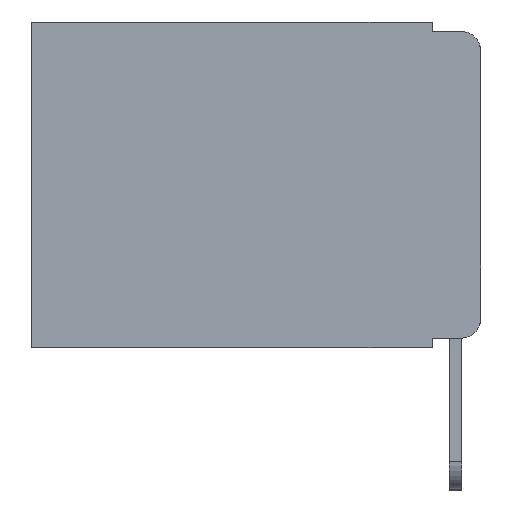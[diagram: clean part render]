
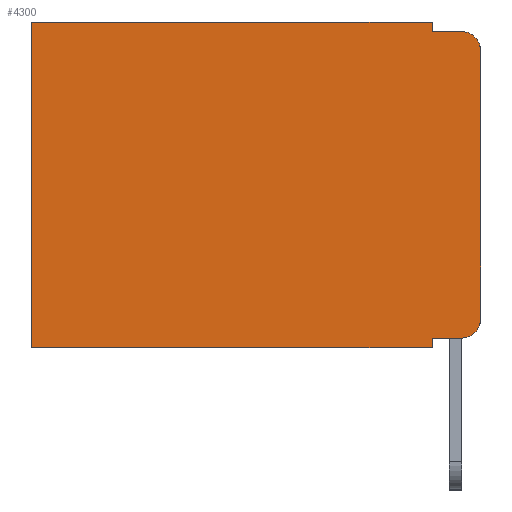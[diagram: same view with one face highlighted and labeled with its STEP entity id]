
A CAD part, left-side view. The second image highlights one B-rep face of the part: STEP entity #4300.
In plain terms, the highlighted planar face has unit normal (-1, 0, 0).
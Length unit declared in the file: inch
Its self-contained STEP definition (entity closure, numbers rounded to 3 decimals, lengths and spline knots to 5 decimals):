
#164 = EDGE_CURVE ( 'NONE', #15296, #22879, #1256, .T. ) ;
#777 = VERTEX_POINT ( 'NONE', #16168 ) ;
#849 = DIRECTION ( 'NONE',  ( 0., 0., -1. ) ) ;
#1256 = CIRCLE ( 'NONE', #5883, 0.02 ) ;
#1416 = ORIENTED_EDGE ( 'NONE', *, *, #164, .T. ) ;
#1510 = VERTEX_POINT ( 'NONE', #14155 ) ;
#1561 = ORIENTED_EDGE ( 'NONE', *, *, #21444, .F. ) ;
#1682 = DIRECTION ( 'NONE',  ( 0., 0., -1. ) ) ;
#1694 = CARTESIAN_POINT ( 'NONE',  ( 0.298, 0., -0.343 ) ) ;
#1709 = CIRCLE ( 'NONE', #3856, 0.02 ) ;
#2006 = EDGE_CURVE ( 'NONE', #1510, #4283, #5034, .T. ) ;
#2026 = VERTEX_POINT ( 'NONE', #12445 ) ;
#2494 = EDGE_CURVE ( 'NONE', #18957, #16139, #8361, .T. ) ;
#2619 = CARTESIAN_POINT ( 'NONE',  ( 0.298, 0.051, -0.333 ) ) ;
#3323 = DIRECTION ( 'NONE',  ( 0., 1., 0. ) ) ;
#3759 = CARTESIAN_POINT ( 'NONE',  ( 0.298, 0., 0. ) ) ;
#3856 = AXIS2_PLACEMENT_3D ( 'NONE', #24052, #13098, #1682 ) ;
#4224 = LINE ( 'NONE', #21386, #13761 ) ;
#4283 = VERTEX_POINT ( 'NONE', #6185 ) ;
#4300 = ADVANCED_FACE ( 'NONE', ( #16237 ), #23213, .F. ) ;
#4496 = LINE ( 'NONE', #1694, #18894 ) ;
#4603 = CARTESIAN_POINT ( 'NONE',  ( 0.298, 0.051, 0. ) ) ;
#4742 = LINE ( 'NONE', #4603, #18541 ) ;
#4749 = CARTESIAN_POINT ( 'NONE',  ( 0.298, 0.02, -0.313 ) ) ;
#4922 = EDGE_CURVE ( 'NONE', #18957, #15296, #13359, .T. ) ;
#5034 = LINE ( 'NONE', #3759, #14545 ) ;
#5145 = DIRECTION ( 'NONE',  ( 0., 0., -1. ) ) ;
#5883 = AXIS2_PLACEMENT_3D ( 'NONE', #4749, #16688, #16767 ) ;
#6026 = DIRECTION ( 'NONE',  ( 1., 0., 0. ) ) ;
#6163 = DIRECTION ( 'NONE',  ( 0., 0., -1. ) ) ;
#6185 = CARTESIAN_POINT ( 'NONE',  ( 0.298, 0.473, 0. ) ) ;
#6301 = CARTESIAN_POINT ( 'NONE',  ( 0.298, 0.02, -0.01 ) ) ;
#6323 = DIRECTION ( 'NONE',  ( 0., 1., 0. ) ) ;
#6912 = AXIS2_PLACEMENT_3D ( 'NONE', #14795, #6026, #6163 ) ;
#6964 = VECTOR ( 'NONE', #23425, 39.37008 ) ;
#7570 = LINE ( 'NONE', #10543, #6964 ) ;
#7580 = DIRECTION ( 'NONE',  ( 0., -1., 0. ) ) ;
#7673 = EDGE_CURVE ( 'NONE', #2026, #23651, #4224, .T. ) ;
#7700 = LINE ( 'NONE', #18250, #12723 ) ;
#8173 = ORIENTED_EDGE ( 'NONE', *, *, #2006, .T. ) ;
#8288 = EDGE_CURVE ( 'NONE', #16139, #19337, #4496, .T. ) ;
#8361 = LINE ( 'NONE', #8645, #17631 ) ;
#8419 = ORIENTED_EDGE ( 'NONE', *, *, #8288, .F. ) ;
#8645 = CARTESIAN_POINT ( 'NONE',  ( 0.298, 0.051, 0. ) ) ;
#8699 = CARTESIAN_POINT ( 'NONE',  ( 0.298, 0.02, -0.333 ) ) ;
#8938 = VECTOR ( 'NONE', #7580, 39.37008 ) ;
#10013 = DIRECTION ( 'NONE',  ( 0., 0., -1. ) ) ;
#10543 = CARTESIAN_POINT ( 'NONE',  ( 0.298, 0., 0. ) ) ;
#11507 = ORIENTED_EDGE ( 'NONE', *, *, #2494, .F. ) ;
#11787 = EDGE_CURVE ( 'NONE', #1510, #2026, #4742, .T. ) ;
#12445 = CARTESIAN_POINT ( 'NONE',  ( 0.298, 0.051, -0.01 ) ) ;
#12723 = VECTOR ( 'NONE', #5145, 39.37008 ) ;
#13087 = ORIENTED_EDGE ( 'NONE', *, *, #4922, .T. ) ;
#13098 = DIRECTION ( 'NONE',  ( -1., 0., 0. ) ) ;
#13359 = LINE ( 'NONE', #13685, #8938 ) ;
#13685 = CARTESIAN_POINT ( 'NONE',  ( 0.298, 0.051, -0.333 ) ) ;
#13761 = VECTOR ( 'NONE', #16219, 39.37008 ) ;
#14155 = CARTESIAN_POINT ( 'NONE',  ( 0.298, 0.051, 0. ) ) ;
#14545 = VECTOR ( 'NONE', #3323, 39.37008 ) ;
#14665 = ORIENTED_EDGE ( 'NONE', *, *, #7673, .F. ) ;
#14795 = CARTESIAN_POINT ( 'NONE',  ( 0.298, 0., 0. ) ) ;
#14924 = EDGE_LOOP ( 'NONE', ( #1561, #19891, #14665, #15191, #8173, #20342, #8419, #11507, #13087, #1416 ) ) ;
#15191 = ORIENTED_EDGE ( 'NONE', *, *, #11787, .F. ) ;
#15296 = VERTEX_POINT ( 'NONE', #8699 ) ;
#16139 = VERTEX_POINT ( 'NONE', #21701 ) ;
#16168 = CARTESIAN_POINT ( 'NONE',  ( 0.298, 0., -0.03 ) ) ;
#16219 = DIRECTION ( 'NONE',  ( 0., -1., 0. ) ) ;
#16237 = FACE_OUTER_BOUND ( 'NONE', #14924, .T. ) ;
#16688 = DIRECTION ( 'NONE',  ( -1., 0., 0. ) ) ;
#16767 = DIRECTION ( 'NONE',  ( 0., 0., -1. ) ) ;
#17631 = VECTOR ( 'NONE', #10013, 39.37008 ) ;
#18214 = EDGE_CURVE ( 'NONE', #777, #23651, #1709, .T. ) ;
#18250 = CARTESIAN_POINT ( 'NONE',  ( 0.298, 0.473, 0. ) ) ;
#18541 = VECTOR ( 'NONE', #849, 39.37008 ) ;
#18625 = CARTESIAN_POINT ( 'NONE',  ( 0.298, 0., -0.313 ) ) ;
#18894 = VECTOR ( 'NONE', #6323, 39.37008 ) ;
#18957 = VERTEX_POINT ( 'NONE', #2619 ) ;
#19337 = VERTEX_POINT ( 'NONE', #22502 ) ;
#19891 = ORIENTED_EDGE ( 'NONE', *, *, #18214, .T. ) ;
#20342 = ORIENTED_EDGE ( 'NONE', *, *, #23942, .T. ) ;
#21386 = CARTESIAN_POINT ( 'NONE',  ( 0.298, 0.051, -0.01 ) ) ;
#21444 = EDGE_CURVE ( 'NONE', #777, #22879, #7570, .T. ) ;
#21701 = CARTESIAN_POINT ( 'NONE',  ( 0.298, 0.051, -0.343 ) ) ;
#22502 = CARTESIAN_POINT ( 'NONE',  ( 0.298, 0.473, -0.343 ) ) ;
#22879 = VERTEX_POINT ( 'NONE', #18625 ) ;
#23213 = PLANE ( 'NONE',  #6912 ) ;
#23425 = DIRECTION ( 'NONE',  ( 0., 0., -1. ) ) ;
#23651 = VERTEX_POINT ( 'NONE', #6301 ) ;
#23942 = EDGE_CURVE ( 'NONE', #4283, #19337, #7700, .T. ) ;
#24052 = CARTESIAN_POINT ( 'NONE',  ( 0.298, 0.02, -0.03 ) ) ;
